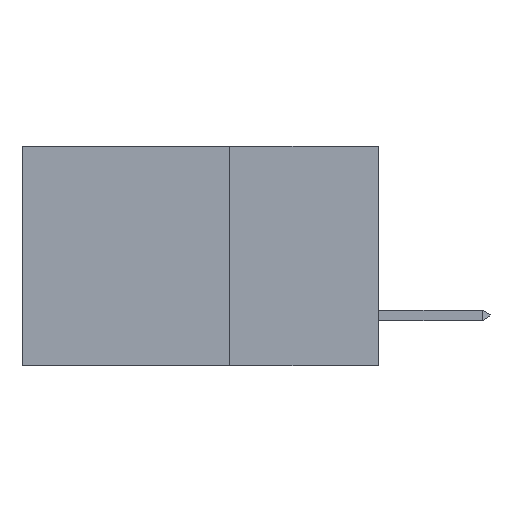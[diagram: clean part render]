
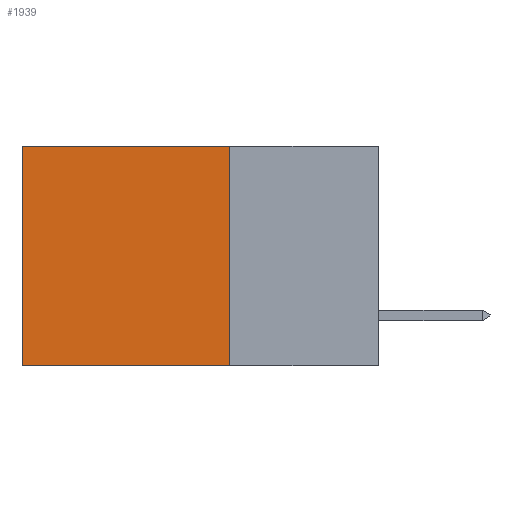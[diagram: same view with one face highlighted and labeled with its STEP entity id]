
A CAD part, left-side view. The second image highlights one B-rep face of the part: STEP entity #1939.
In plain terms, the highlighted planar face has unit normal (-1, 0, 0).
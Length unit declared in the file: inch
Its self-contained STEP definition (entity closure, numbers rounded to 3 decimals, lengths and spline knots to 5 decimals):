
#426 = CARTESIAN_POINT ( 'NONE',  ( 0.298, 0.6, 0. ) ) ;
#527 = EDGE_CURVE ( 'NONE', #3009, #4912, #4955, .T. ) ;
#629 = VERTEX_POINT ( 'NONE', #13504 ) ;
#644 = LINE ( 'NONE', #14319, #8816 ) ;
#663 = CARTESIAN_POINT ( 'NONE',  ( 0.298, 0.25, 0. ) ) ;
#942 = VERTEX_POINT ( 'NONE', #663 ) ;
#1113 = EDGE_CURVE ( 'NONE', #629, #4912, #8103, .T. ) ;
#1939 = ADVANCED_FACE ( 'NONE', ( #3419 ), #5832, .F. ) ;
#2891 = EDGE_CURVE ( 'NONE', #942, #3009, #3022, .T. ) ;
#3009 = VERTEX_POINT ( 'NONE', #10265 ) ;
#3022 = LINE ( 'NONE', #13349, #11562 ) ;
#3307 = VECTOR ( 'NONE', #11012, 39.37008 ) ;
#3419 = FACE_OUTER_BOUND ( 'NONE', #9791, .T. ) ;
#4912 = VERTEX_POINT ( 'NONE', #5521 ) ;
#4955 = LINE ( 'NONE', #426, #3307 ) ;
#5038 = DIRECTION ( 'NONE',  ( 1., 0., 0. ) ) ;
#5521 = CARTESIAN_POINT ( 'NONE',  ( 0.298, 0.6, -0.37 ) ) ;
#5832 = PLANE ( 'NONE',  #8472 ) ;
#5908 = ORIENTED_EDGE ( 'NONE', *, *, #527, .T. ) ;
#6259 = DIRECTION ( 'NONE',  ( 0., 1., 0. ) ) ;
#8082 = ORIENTED_EDGE ( 'NONE', *, *, #14175, .F. ) ;
#8103 = LINE ( 'NONE', #10568, #15161 ) ;
#8392 = ORIENTED_EDGE ( 'NONE', *, *, #2891, .T. ) ;
#8472 = AXIS2_PLACEMENT_3D ( 'NONE', #12328, #5038, #13370 ) ;
#8816 = VECTOR ( 'NONE', #10706, 39.37008 ) ;
#9791 = EDGE_LOOP ( 'NONE', ( #5908, #10686, #8082, #8392 ) ) ;
#10265 = CARTESIAN_POINT ( 'NONE',  ( 0.298, 0.6, 0. ) ) ;
#10568 = CARTESIAN_POINT ( 'NONE',  ( 0.298, 0.25, -0.37 ) ) ;
#10686 = ORIENTED_EDGE ( 'NONE', *, *, #1113, .F. ) ;
#10706 = DIRECTION ( 'NONE',  ( 0., 0., -1. ) ) ;
#11012 = DIRECTION ( 'NONE',  ( 0., 0., -1. ) ) ;
#11562 = VECTOR ( 'NONE', #6259, 39.37008 ) ;
#12328 = CARTESIAN_POINT ( 'NONE',  ( 0.298, 0.25, 0. ) ) ;
#12971 = DIRECTION ( 'NONE',  ( 0., 1., 0. ) ) ;
#13349 = CARTESIAN_POINT ( 'NONE',  ( 0.298, 0.25, 0. ) ) ;
#13370 = DIRECTION ( 'NONE',  ( 0., 0., -1. ) ) ;
#13504 = CARTESIAN_POINT ( 'NONE',  ( 0.298, 0.25, -0.37 ) ) ;
#14175 = EDGE_CURVE ( 'NONE', #942, #629, #644, .T. ) ;
#14319 = CARTESIAN_POINT ( 'NONE',  ( 0.298, 0.25, 0. ) ) ;
#15161 = VECTOR ( 'NONE', #12971, 39.37008 ) ;
